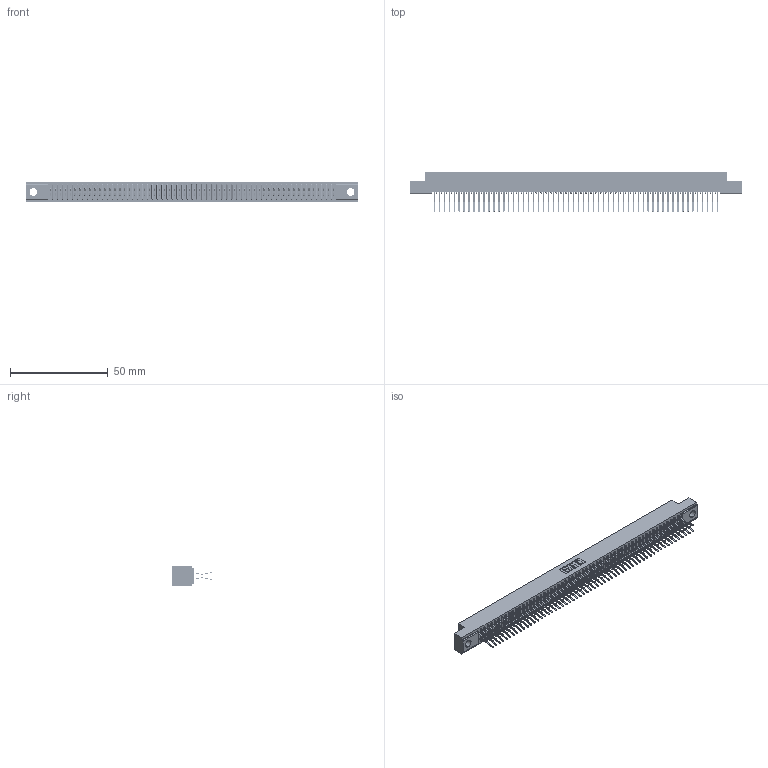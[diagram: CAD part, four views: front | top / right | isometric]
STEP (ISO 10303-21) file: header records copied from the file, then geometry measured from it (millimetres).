
FILE_DESCRIPTION (( 'STEP AP203' ), '1' );
FILE_NAME ('391-116-560-204.STEP', '2018-08-09T23:27:44', ( '' ), ( '' ), 'SwSTEP 2.0', 'SolidWorks 2016', '' );
FILE_SCHEMA (( 'CONFIG_CONTROL_DESIGN' ));
Length unit declared in the file: inch
Products named in the file (3): 391-116-560-204; 341 Part_.156 (3.96) Dia Mounting Holes; 341-292-001_341-292-160
Assembly tree (117 placements, depth 2):
  391-116-560-204
    341 Part_.156 (3.96) Dia Mounting Holes
    341-292-001_341-292-160  x116
Bounding box: 169.54 x 20.37 x 10.16 mm (x, y, z)
Volume: 12543.4 mm3; surface area: 23516.2 mm2
Topology: 117 solids, 117 shells, 8250 faces, 23958 edges, 15542 vertices
Faces by surface type: plane 4722, cylinder 3296, sphere 118, torus 114
Entity records: 68619 total; most frequent: CARTESIAN_POINT 11412, ORIENTED_EDGE 11340, DIRECTION 11060, EDGE_CURVE 5670, VECTOR 4600, LINE 4600, VERTEX_POINT 3582, AXIS2_PLACEMENT_3D 3230
